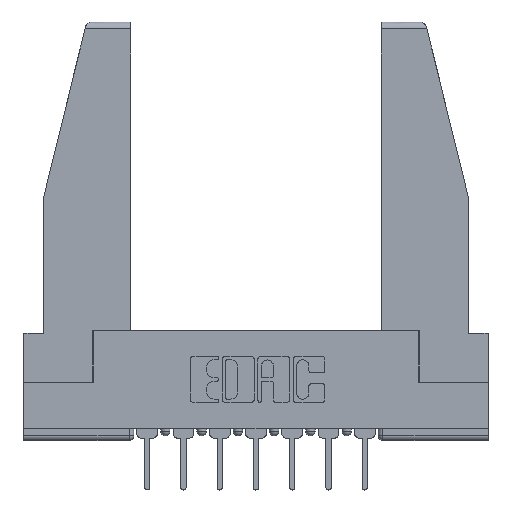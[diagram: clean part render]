
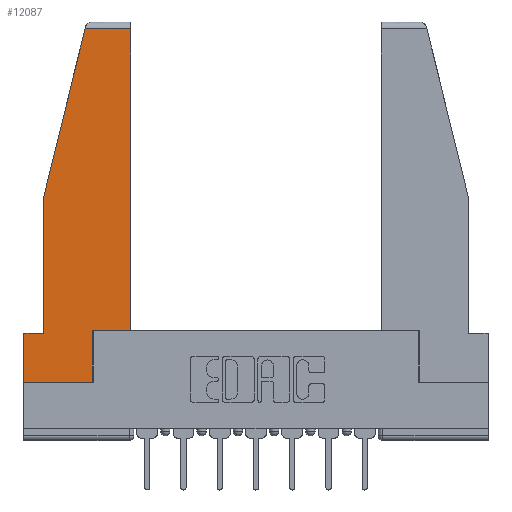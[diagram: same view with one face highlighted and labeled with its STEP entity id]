
A CAD part, top view. The second image highlights one B-rep face of the part: STEP entity #12087.
In plain terms, the highlighted planar face has unit normal (0, 0, 1).
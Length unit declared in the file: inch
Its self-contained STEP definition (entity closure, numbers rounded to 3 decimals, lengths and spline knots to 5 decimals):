
#39 = EDGE_CURVE ( 'NONE', #4928, #3706, #5284, .T. ) ;
#412 = LINE ( 'NONE', #11175, #2829 ) ;
#547 = LINE ( 'NONE', #4576, #9912 ) ;
#577 = DIRECTION ( 'NONE',  ( 0., -1., 0. ) ) ;
#785 = CARTESIAN_POINT ( 'NONE',  ( 0.297, 0.223, 0. ) ) ;
#897 = EDGE_CURVE ( 'NONE', #7287, #3864, #11278, .T. ) ;
#1167 = FACE_OUTER_BOUND ( 'NONE', #5207, .T. ) ;
#1286 = CARTESIAN_POINT ( 'NONE',  ( 0.461, 0.223, 0. ) ) ;
#1328 = CARTESIAN_POINT ( 'NONE',  ( 0., 0., 0. ) ) ;
#1550 = LINE ( 'NONE', #4721, #12094 ) ;
#1645 = EDGE_CURVE ( 'NONE', #5541, #5486, #547, .T. ) ;
#1774 = VECTOR ( 'NONE', #4680, 39.37008 ) ;
#1853 = ORIENTED_EDGE ( 'NONE', *, *, #7495, .T. ) ;
#2167 = CARTESIAN_POINT ( 'NONE',  ( 0., 1.52, 0. ) ) ;
#2197 = CARTESIAN_POINT ( 'NONE',  ( 0., 0.21, 0. ) ) ;
#2300 = DIRECTION ( 'NONE',  ( -1., 0., 0. ) ) ;
#2595 = DIRECTION ( 'NONE',  ( 0., 1., 0. ) ) ;
#2712 = CARTESIAN_POINT ( 'NONE',  ( 0.271, 1.55, 0. ) ) ;
#2829 = VECTOR ( 'NONE', #6207, 39.37008 ) ;
#3024 = VERTEX_POINT ( 'NONE', #6223 ) ;
#3258 = VECTOR ( 'NONE', #5347, 39.37008 ) ;
#3706 = VERTEX_POINT ( 'NONE', #4867 ) ;
#3864 = VERTEX_POINT ( 'NONE', #4225 ) ;
#4225 = CARTESIAN_POINT ( 'NONE',  ( 0.2636, 1.52, 0. ) ) ;
#4434 = DIRECTION ( 'NONE',  ( -1., 0., 0. ) ) ;
#4576 = CARTESIAN_POINT ( 'NONE',  ( 0.297, 0., 0. ) ) ;
#4680 = DIRECTION ( 'NONE',  ( -0.239, -0.971, 0. ) ) ;
#4721 = CARTESIAN_POINT ( 'NONE',  ( 0.461, 0.223, 0. ) ) ;
#4867 = CARTESIAN_POINT ( 'NONE',  ( 0., 0.21, 0. ) ) ;
#4928 = VERTEX_POINT ( 'NONE', #5349 ) ;
#5207 = EDGE_LOOP ( 'NONE', ( #12003, #12025, #9586, #7020, #7066, #9035, #1853, #5712, #11959 ) ) ;
#5245 = EDGE_CURVE ( 'NONE', #3706, #3024, #7372, .T. ) ;
#5284 = LINE ( 'NONE', #2197, #10548 ) ;
#5347 = DIRECTION ( 'NONE',  ( 1., 0., 0. ) ) ;
#5349 = CARTESIAN_POINT ( 'NONE',  ( 0.086, 0.21, 0. ) ) ;
#5486 = VERTEX_POINT ( 'NONE', #785 ) ;
#5541 = VERTEX_POINT ( 'NONE', #12661 ) ;
#5712 = ORIENTED_EDGE ( 'NONE', *, *, #1645, .T. ) ;
#5862 = PLANE ( 'NONE',  #8559 ) ;
#6109 = CARTESIAN_POINT ( 'NONE',  ( 0.086, 0.8, 0. ) ) ;
#6207 = DIRECTION ( 'NONE',  ( 1., 0., 0. ) ) ;
#6223 = CARTESIAN_POINT ( 'NONE',  ( 0., 0., 0. ) ) ;
#6284 = CARTESIAN_POINT ( 'NONE',  ( 0.086, 0.8, 0. ) ) ;
#6338 = LINE ( 'NONE', #1328, #3258 ) ;
#7020 = ORIENTED_EDGE ( 'NONE', *, *, #8700, .T. ) ;
#7066 = ORIENTED_EDGE ( 'NONE', *, *, #39, .T. ) ;
#7287 = VERTEX_POINT ( 'NONE', #10924 ) ;
#7372 = LINE ( 'NONE', #9328, #9842 ) ;
#7373 = EDGE_CURVE ( 'NONE', #5486, #12640, #412, .T. ) ;
#7495 = EDGE_CURVE ( 'NONE', #3024, #5541, #6338, .T. ) ;
#7535 = EDGE_CURVE ( 'NONE', #3864, #10170, #9720, .T. ) ;
#7875 = VECTOR ( 'NONE', #2300, 39.37008 ) ;
#7895 = DIRECTION ( 'NONE',  ( 0., 0., 1. ) ) ;
#8435 = LINE ( 'NONE', #6284, #12295 ) ;
#8559 = AXIS2_PLACEMENT_3D ( 'NONE', #9859, #7895, #10226 ) ;
#8700 = EDGE_CURVE ( 'NONE', #10170, #4928, #8435, .T. ) ;
#9035 = ORIENTED_EDGE ( 'NONE', *, *, #5245, .T. ) ;
#9328 = CARTESIAN_POINT ( 'NONE',  ( 0., 0.21, 0. ) ) ;
#9586 = ORIENTED_EDGE ( 'NONE', *, *, #7535, .T. ) ;
#9720 = LINE ( 'NONE', #2712, #1774 ) ;
#9810 = EDGE_CURVE ( 'NONE', #12640, #7287, #1550, .T. ) ;
#9842 = VECTOR ( 'NONE', #577, 39.37008 ) ;
#9859 = CARTESIAN_POINT ( 'NONE',  ( 0., 0., 0. ) ) ;
#9912 = VECTOR ( 'NONE', #2595, 39.37008 ) ;
#10170 = VERTEX_POINT ( 'NONE', #6109 ) ;
#10226 = DIRECTION ( 'NONE',  ( 1., 0., 0. ) ) ;
#10548 = VECTOR ( 'NONE', #4434, 39.37008 ) ;
#10924 = CARTESIAN_POINT ( 'NONE',  ( 0.461, 1.52, 0. ) ) ;
#11175 = CARTESIAN_POINT ( 'NONE',  ( 0.297, 0.223, 0. ) ) ;
#11278 = LINE ( 'NONE', #2167, #7875 ) ;
#11659 = DIRECTION ( 'NONE',  ( 0., 1., 0. ) ) ;
#11959 = ORIENTED_EDGE ( 'NONE', *, *, #7373, .T. ) ;
#12003 = ORIENTED_EDGE ( 'NONE', *, *, #9810, .T. ) ;
#12025 = ORIENTED_EDGE ( 'NONE', *, *, #897, .T. ) ;
#12087 = ADVANCED_FACE ( 'NONE', ( #1167 ), #5862, .T. ) ;
#12094 = VECTOR ( 'NONE', #11659, 39.37008 ) ;
#12295 = VECTOR ( 'NONE', #12305, 39.37008 ) ;
#12305 = DIRECTION ( 'NONE',  ( 0., -1., 0. ) ) ;
#12640 = VERTEX_POINT ( 'NONE', #1286 ) ;
#12661 = CARTESIAN_POINT ( 'NONE',  ( 0.297, 0., 0. ) ) ;
